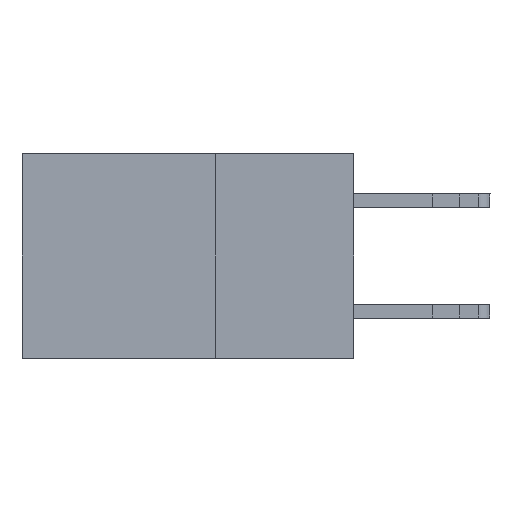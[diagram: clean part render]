
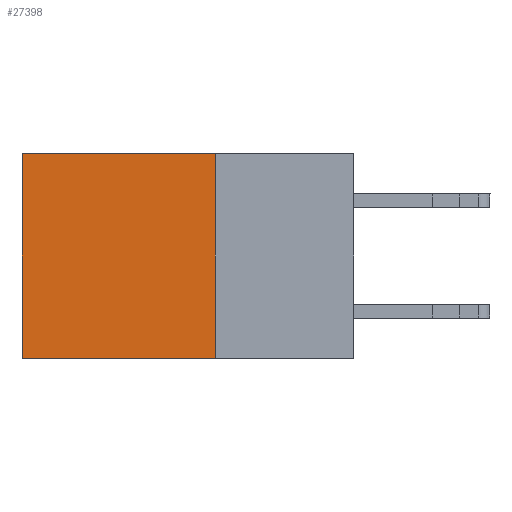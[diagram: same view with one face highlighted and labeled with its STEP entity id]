
A CAD part, left-side view. The second image highlights one B-rep face of the part: STEP entity #27398.
In plain terms, the highlighted planar face has unit normal (-1, 0, 0).
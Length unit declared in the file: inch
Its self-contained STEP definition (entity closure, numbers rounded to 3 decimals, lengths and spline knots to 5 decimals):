
#129 = LINE ( 'NONE', #3673, #1394 ) ;
#273 = DIRECTION ( 'NONE',  ( 0., 1., 0. ) ) ;
#1394 = VECTOR ( 'NONE', #11703, 39.37008 ) ;
#1444 = ORIENTED_EDGE ( 'NONE', *, *, #28675, .F. ) ;
#1869 = EDGE_CURVE ( 'NONE', #8867, #16219, #16210, .T. ) ;
#2476 = CARTESIAN_POINT ( 'NONE',  ( 0.2875, 0.25, 0. ) ) ;
#3263 = AXIS2_PLACEMENT_3D ( 'NONE', #31869, #10712, #16106 ) ;
#3673 = CARTESIAN_POINT ( 'NONE',  ( 0.2875, 0.6, 0. ) ) ;
#5749 = VECTOR ( 'NONE', #13706, 39.37008 ) ;
#5846 = CARTESIAN_POINT ( 'NONE',  ( 0.2875, 0.6, -0.37 ) ) ;
#7676 = DIRECTION ( 'NONE',  ( 0., 1., 0. ) ) ;
#8467 = ORIENTED_EDGE ( 'NONE', *, *, #25461, .T. ) ;
#8867 = VERTEX_POINT ( 'NONE', #22007 ) ;
#10712 = DIRECTION ( 'NONE',  ( 1., 0., 0. ) ) ;
#10784 = EDGE_LOOP ( 'NONE', ( #8467, #1444, #27762, #33883 ) ) ;
#11703 = DIRECTION ( 'NONE',  ( 0., 0., -1. ) ) ;
#12977 = EDGE_CURVE ( 'NONE', #8867, #21517, #13401, .T. ) ;
#13401 = LINE ( 'NONE', #2476, #26624 ) ;
#13706 = DIRECTION ( 'NONE',  ( 0., 0., -1. ) ) ;
#14463 = VERTEX_POINT ( 'NONE', #5846 ) ;
#15861 = PLANE ( 'NONE',  #3263 ) ;
#16106 = DIRECTION ( 'NONE',  ( 0., 0., -1. ) ) ;
#16210 = LINE ( 'NONE', #21089, #5749 ) ;
#16219 = VERTEX_POINT ( 'NONE', #33983 ) ;
#20018 = LINE ( 'NONE', #23579, #25782 ) ;
#20708 = CARTESIAN_POINT ( 'NONE',  ( 0.2875, 0.6, 0. ) ) ;
#20746 = FACE_OUTER_BOUND ( 'NONE', #10784, .T. ) ;
#21089 = CARTESIAN_POINT ( 'NONE',  ( 0.2875, 0.25, 0. ) ) ;
#21517 = VERTEX_POINT ( 'NONE', #20708 ) ;
#22007 = CARTESIAN_POINT ( 'NONE',  ( 0.2875, 0.25, 0. ) ) ;
#23579 = CARTESIAN_POINT ( 'NONE',  ( 0.2875, 0.25, -0.37 ) ) ;
#25461 = EDGE_CURVE ( 'NONE', #21517, #14463, #129, .T. ) ;
#25782 = VECTOR ( 'NONE', #7676, 39.37008 ) ;
#26624 = VECTOR ( 'NONE', #273, 39.37008 ) ;
#27398 = ADVANCED_FACE ( 'NONE', ( #20746 ), #15861, .F. ) ;
#27762 = ORIENTED_EDGE ( 'NONE', *, *, #1869, .F. ) ;
#28675 = EDGE_CURVE ( 'NONE', #16219, #14463, #20018, .T. ) ;
#31869 = CARTESIAN_POINT ( 'NONE',  ( 0.2875, 0.25, 0. ) ) ;
#33883 = ORIENTED_EDGE ( 'NONE', *, *, #12977, .T. ) ;
#33983 = CARTESIAN_POINT ( 'NONE',  ( 0.2875, 0.25, -0.37 ) ) ;
